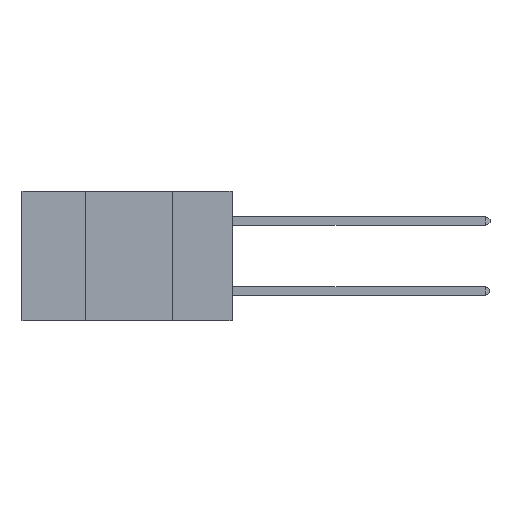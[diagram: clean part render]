
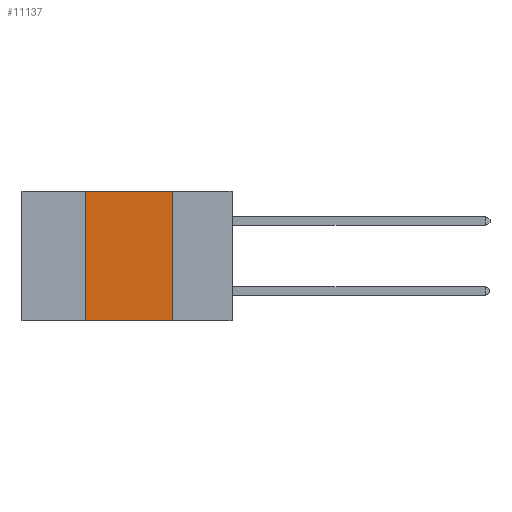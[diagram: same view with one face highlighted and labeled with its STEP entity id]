
A CAD part, left-side view. The second image highlights one B-rep face of the part: STEP entity #11137.
In plain terms, the highlighted planar face has unit normal (-1, 0, 0).
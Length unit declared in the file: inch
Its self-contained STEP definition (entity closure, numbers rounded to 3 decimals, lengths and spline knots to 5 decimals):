
#41 = CARTESIAN_POINT ( 'NONE',  ( 0., 0.42, 0. ) ) ;
#764 = CARTESIAN_POINT ( 'NONE',  ( 0., 0.6, 0. ) ) ;
#850 = LINE ( 'NONE', #2157, #15158 ) ;
#1544 = CARTESIAN_POINT ( 'NONE',  ( 0., 0.17, 0. ) ) ;
#2157 = CARTESIAN_POINT ( 'NONE',  ( 0., 0.6, 0. ) ) ;
#2848 = CARTESIAN_POINT ( 'NONE',  ( 0., 0.6, -0.37 ) ) ;
#3135 = DIRECTION ( 'NONE',  ( 0., 0., -1. ) ) ;
#3294 = VERTEX_POINT ( 'NONE', #5467 ) ;
#4023 = DIRECTION ( 'NONE',  ( 0., 0., -1. ) ) ;
#4888 = VERTEX_POINT ( 'NONE', #14346 ) ;
#5226 = VERTEX_POINT ( 'NONE', #7200 ) ;
#5442 = PLANE ( 'NONE',  #10276 ) ;
#5467 = CARTESIAN_POINT ( 'NONE',  ( 0., 0.42, 0. ) ) ;
#5655 = CARTESIAN_POINT ( 'NONE',  ( 0., 0.42, -0.37 ) ) ;
#6195 = LINE ( 'NONE', #1544, #12778 ) ;
#7200 = CARTESIAN_POINT ( 'NONE',  ( 0., 0.17, 0. ) ) ;
#7221 = FACE_OUTER_BOUND ( 'NONE', #13312, .T. ) ;
#7359 = EDGE_CURVE ( 'NONE', #14421, #3294, #10466, .T. ) ;
#7363 = VECTOR ( 'NONE', #10166, 39.37008 ) ;
#8092 = DIRECTION ( 'NONE',  ( 0., -1., 0. ) ) ;
#10166 = DIRECTION ( 'NONE',  ( 0., 0., 1. ) ) ;
#10276 = AXIS2_PLACEMENT_3D ( 'NONE', #764, #12162, #4023 ) ;
#10466 = LINE ( 'NONE', #41, #7363 ) ;
#10744 = ORIENTED_EDGE ( 'NONE', *, *, #13296, .F. ) ;
#11137 = ADVANCED_FACE ( 'NONE', ( #7221 ), #5442, .F. ) ;
#11145 = ORIENTED_EDGE ( 'NONE', *, *, #7359, .F. ) ;
#11169 = LINE ( 'NONE', #2848, #14646 ) ;
#11693 = EDGE_CURVE ( 'NONE', #3294, #5226, #850, .T. ) ;
#12162 = DIRECTION ( 'NONE',  ( 1., 0., 0. ) ) ;
#12778 = VECTOR ( 'NONE', #3135, 39.37008 ) ;
#13296 = EDGE_CURVE ( 'NONE', #5226, #4888, #6195, .T. ) ;
#13312 = EDGE_LOOP ( 'NONE', ( #10744, #14201, #11145, #14622 ) ) ;
#13736 = DIRECTION ( 'NONE',  ( 0., -1., 0. ) ) ;
#13859 = EDGE_CURVE ( 'NONE', #14421, #4888, #11169, .T. ) ;
#14201 = ORIENTED_EDGE ( 'NONE', *, *, #11693, .F. ) ;
#14346 = CARTESIAN_POINT ( 'NONE',  ( 0., 0.17, -0.37 ) ) ;
#14421 = VERTEX_POINT ( 'NONE', #5655 ) ;
#14622 = ORIENTED_EDGE ( 'NONE', *, *, #13859, .T. ) ;
#14646 = VECTOR ( 'NONE', #13736, 39.37008 ) ;
#15158 = VECTOR ( 'NONE', #8092, 39.37008 ) ;
